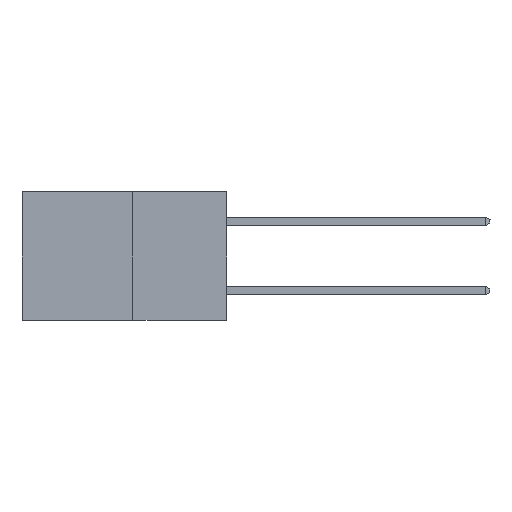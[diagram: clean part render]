
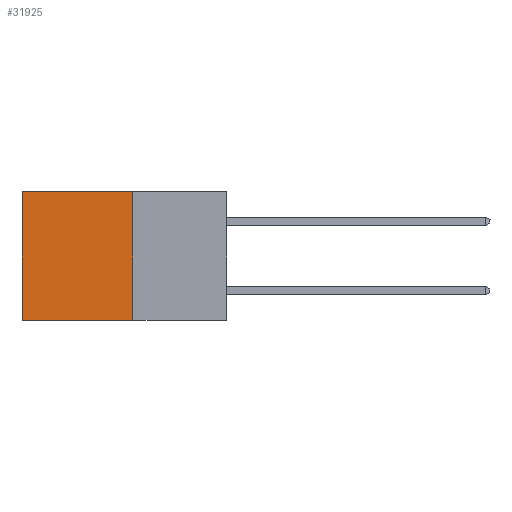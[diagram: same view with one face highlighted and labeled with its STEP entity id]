
A CAD part, left-side view. The second image highlights one B-rep face of the part: STEP entity #31925.
In plain terms, the highlighted planar face has unit normal (-1, 0, 0).
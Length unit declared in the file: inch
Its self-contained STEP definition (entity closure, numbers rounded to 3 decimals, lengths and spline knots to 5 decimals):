
#459 = EDGE_CURVE ( 'NONE', #33327, #8452, #8458, .T. ) ;
#921 = FACE_OUTER_BOUND ( 'NONE', #29457, .T. ) ;
#2340 = VECTOR ( 'NONE', #27018, 39.37008 ) ;
#3074 = VECTOR ( 'NONE', #32393, 39.37008 ) ;
#3991 = EDGE_CURVE ( 'NONE', #8291, #33327, #31031, .T. ) ;
#8291 = VERTEX_POINT ( 'NONE', #13429 ) ;
#8408 = PLANE ( 'NONE',  #32014 ) ;
#8452 = VERTEX_POINT ( 'NONE', #8636 ) ;
#8458 = LINE ( 'NONE', #32050, #3074 ) ;
#8517 = ORIENTED_EDGE ( 'NONE', *, *, #22138, .F. ) ;
#8636 = CARTESIAN_POINT ( 'NONE',  ( 0.277, 0.59, -0.37 ) ) ;
#10059 = DIRECTION ( 'NONE',  ( 0., 1., 0. ) ) ;
#10295 = CARTESIAN_POINT ( 'NONE',  ( 0.277, 0.27, 0. ) ) ;
#10794 = CARTESIAN_POINT ( 'NONE',  ( 0.277, 0.59, 0. ) ) ;
#10852 = VECTOR ( 'NONE', #33767, 39.37008 ) ;
#11092 = DIRECTION ( 'NONE',  ( 1., 0., 0. ) ) ;
#12742 = CARTESIAN_POINT ( 'NONE',  ( 0.277, 0.27, -0.37 ) ) ;
#13429 = CARTESIAN_POINT ( 'NONE',  ( 0.277, 0.27, 0. ) ) ;
#16493 = LINE ( 'NONE', #24396, #2340 ) ;
#21716 = ORIENTED_EDGE ( 'NONE', *, *, #28728, .F. ) ;
#22138 = EDGE_CURVE ( 'NONE', #27816, #8452, #31860, .T. ) ;
#23285 = VECTOR ( 'NONE', #10059, 39.37008 ) ;
#24044 = ORIENTED_EDGE ( 'NONE', *, *, #459, .T. ) ;
#24396 = CARTESIAN_POINT ( 'NONE',  ( 0.277, 0.27, -0.37 ) ) ;
#25941 = CARTESIAN_POINT ( 'NONE',  ( 0.277, 0.27, -0.37 ) ) ;
#26924 = CARTESIAN_POINT ( 'NONE',  ( 0.277, 0.27, -0.37 ) ) ;
#27018 = DIRECTION ( 'NONE',  ( 0., 0., -1. ) ) ;
#27816 = VERTEX_POINT ( 'NONE', #25941 ) ;
#28728 = EDGE_CURVE ( 'NONE', #8291, #27816, #16493, .T. ) ;
#29457 = EDGE_LOOP ( 'NONE', ( #24044, #8517, #21716, #30780 ) ) ;
#29536 = DIRECTION ( 'NONE',  ( 0., 0., -1. ) ) ;
#30780 = ORIENTED_EDGE ( 'NONE', *, *, #3991, .T. ) ;
#31031 = LINE ( 'NONE', #10295, #23285 ) ;
#31860 = LINE ( 'NONE', #12742, #10852 ) ;
#31925 = ADVANCED_FACE ( 'NONE', ( #921 ), #8408, .F. ) ;
#32014 = AXIS2_PLACEMENT_3D ( 'NONE', #26924, #11092, #29536 ) ;
#32050 = CARTESIAN_POINT ( 'NONE',  ( 0.277, 0.59, -0.37 ) ) ;
#32393 = DIRECTION ( 'NONE',  ( 0., 0., -1. ) ) ;
#33327 = VERTEX_POINT ( 'NONE', #10794 ) ;
#33767 = DIRECTION ( 'NONE',  ( 0., 1., 0. ) ) ;
